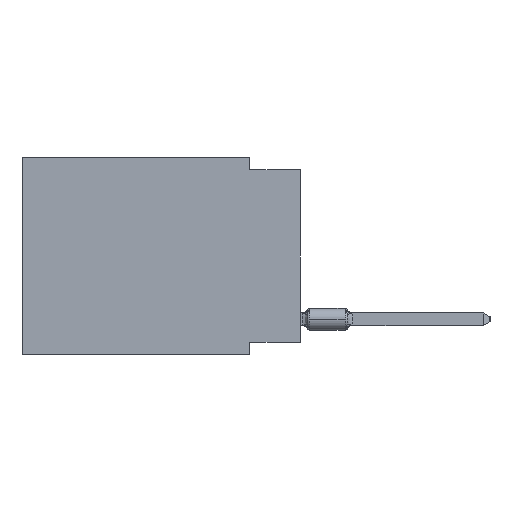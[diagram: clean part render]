
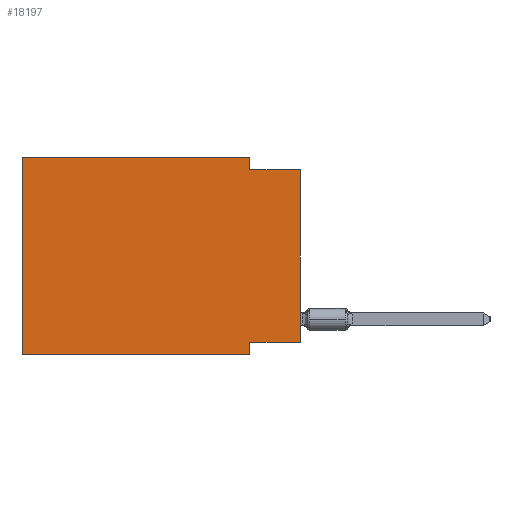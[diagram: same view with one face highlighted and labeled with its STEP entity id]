
A CAD part, left-side view. The second image highlights one B-rep face of the part: STEP entity #18197.
In plain terms, the highlighted planar face has unit normal (-1, 0, 0).
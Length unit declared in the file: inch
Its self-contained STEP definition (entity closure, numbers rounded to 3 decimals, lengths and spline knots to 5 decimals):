
#526 = DIRECTION ( 'NONE',  ( 0., 0., -1. ) ) ;
#918 = DIRECTION ( 'NONE',  ( 0., -1., 0. ) ) ;
#1103 = LINE ( 'NONE', #27260, #4658 ) ;
#1604 = DIRECTION ( 'NONE',  ( 0., 0., -1. ) ) ;
#1804 = VECTOR ( 'NONE', #2026, 39.37008 ) ;
#2026 = DIRECTION ( 'NONE',  ( 0., 0., 1. ) ) ;
#3741 = CARTESIAN_POINT ( 'NONE',  ( 0., 0.1, -0.365 ) ) ;
#3867 = LINE ( 'NONE', #37261, #14551 ) ;
#4135 = LINE ( 'NONE', #32392, #4552 ) ;
#4552 = VECTOR ( 'NONE', #918, 39.37008 ) ;
#4619 = CARTESIAN_POINT ( 'NONE',  ( 0., 0.1, -0.025 ) ) ;
#4658 = VECTOR ( 'NONE', #12673, 39.37008 ) ;
#6732 = VECTOR ( 'NONE', #31387, 39.37008 ) ;
#8755 = CARTESIAN_POINT ( 'NONE',  ( 0., 0., -0.025 ) ) ;
#8945 = EDGE_CURVE ( 'NONE', #18767, #10059, #9689, .T. ) ;
#9159 = EDGE_CURVE ( 'NONE', #25967, #15891, #27864, .T. ) ;
#9689 = LINE ( 'NONE', #36202, #22010 ) ;
#10014 = ORIENTED_EDGE ( 'NONE', *, *, #14386, .F. ) ;
#10042 = AXIS2_PLACEMENT_3D ( 'NONE', #33282, #15838, #1604 ) ;
#10059 = VERTEX_POINT ( 'NONE', #15210 ) ;
#10576 = CARTESIAN_POINT ( 'NONE',  ( 0., 0., -0.365 ) ) ;
#11114 = LINE ( 'NONE', #19632, #6732 ) ;
#12673 = DIRECTION ( 'NONE',  ( 0., 1., 0. ) ) ;
#13175 = FACE_OUTER_BOUND ( 'NONE', #26091, .T. ) ;
#13762 = LINE ( 'NONE', #36877, #1804 ) ;
#14386 = EDGE_CURVE ( 'NONE', #18337, #18767, #11114, .T. ) ;
#14551 = VECTOR ( 'NONE', #23747, 39.37008 ) ;
#15210 = CARTESIAN_POINT ( 'NONE',  ( 0., 0.1, 0. ) ) ;
#15838 = DIRECTION ( 'NONE',  ( 1., 0., 0. ) ) ;
#15891 = VERTEX_POINT ( 'NONE', #8755 ) ;
#16393 = PLANE ( 'NONE',  #10042 ) ;
#17148 = CARTESIAN_POINT ( 'NONE',  ( 0., 0.55, 0. ) ) ;
#17587 = CARTESIAN_POINT ( 'NONE',  ( 0., 0.1, 0. ) ) ;
#17635 = ORIENTED_EDGE ( 'NONE', *, *, #22974, .F. ) ;
#17712 = EDGE_CURVE ( 'NONE', #18337, #29370, #4135, .T. ) ;
#18197 = ADVANCED_FACE ( 'NONE', ( #13175 ), #16393, .F. ) ;
#18337 = VERTEX_POINT ( 'NONE', #37041 ) ;
#18767 = VERTEX_POINT ( 'NONE', #17148 ) ;
#19632 = CARTESIAN_POINT ( 'NONE',  ( 0., 0.55, 0. ) ) ;
#21355 = EDGE_CURVE ( 'NONE', #10059, #25967, #25919, .T. ) ;
#22010 = VECTOR ( 'NONE', #33003, 39.37008 ) ;
#22168 = DIRECTION ( 'NONE',  ( 0., -1., 0. ) ) ;
#22974 = EDGE_CURVE ( 'NONE', #24053, #32431, #1103, .T. ) ;
#23393 = ORIENTED_EDGE ( 'NONE', *, *, #27862, .T. ) ;
#23747 = DIRECTION ( 'NONE',  ( 0., 0., -1. ) ) ;
#24053 = VERTEX_POINT ( 'NONE', #10576 ) ;
#24141 = ORIENTED_EDGE ( 'NONE', *, *, #8945, .F. ) ;
#24354 = VECTOR ( 'NONE', #526, 39.37008 ) ;
#25330 = ORIENTED_EDGE ( 'NONE', *, *, #17712, .T. ) ;
#25919 = LINE ( 'NONE', #17587, #24354 ) ;
#25967 = VERTEX_POINT ( 'NONE', #4619 ) ;
#26091 = EDGE_LOOP ( 'NONE', ( #23393, #30912, #32164, #24141, #10014, #25330, #29453, #17635 ) ) ;
#27260 = CARTESIAN_POINT ( 'NONE',  ( 0., 0., -0.365 ) ) ;
#27862 = EDGE_CURVE ( 'NONE', #24053, #15891, #13762, .T. ) ;
#27864 = LINE ( 'NONE', #36946, #34753 ) ;
#27945 = EDGE_CURVE ( 'NONE', #32431, #29370, #3867, .T. ) ;
#29370 = VERTEX_POINT ( 'NONE', #31160 ) ;
#29453 = ORIENTED_EDGE ( 'NONE', *, *, #27945, .F. ) ;
#30912 = ORIENTED_EDGE ( 'NONE', *, *, #9159, .F. ) ;
#31160 = CARTESIAN_POINT ( 'NONE',  ( 0., 0.1, -0.39 ) ) ;
#31387 = DIRECTION ( 'NONE',  ( 0., 0., 1. ) ) ;
#32164 = ORIENTED_EDGE ( 'NONE', *, *, #21355, .F. ) ;
#32392 = CARTESIAN_POINT ( 'NONE',  ( 0., 0.55, -0.39 ) ) ;
#32431 = VERTEX_POINT ( 'NONE', #3741 ) ;
#33003 = DIRECTION ( 'NONE',  ( 0., -1., 0. ) ) ;
#33282 = CARTESIAN_POINT ( 'NONE',  ( 0., 0.55, 0. ) ) ;
#34753 = VECTOR ( 'NONE', #22168, 39.37008 ) ;
#36202 = CARTESIAN_POINT ( 'NONE',  ( 0., 0.55, 0. ) ) ;
#36877 = CARTESIAN_POINT ( 'NONE',  ( 0., 0., 0. ) ) ;
#36946 = CARTESIAN_POINT ( 'NONE',  ( 0., 0., -0.025 ) ) ;
#37041 = CARTESIAN_POINT ( 'NONE',  ( 0., 0.55, -0.39 ) ) ;
#37261 = CARTESIAN_POINT ( 'NONE',  ( 0., 0.1, -0.39 ) ) ;
